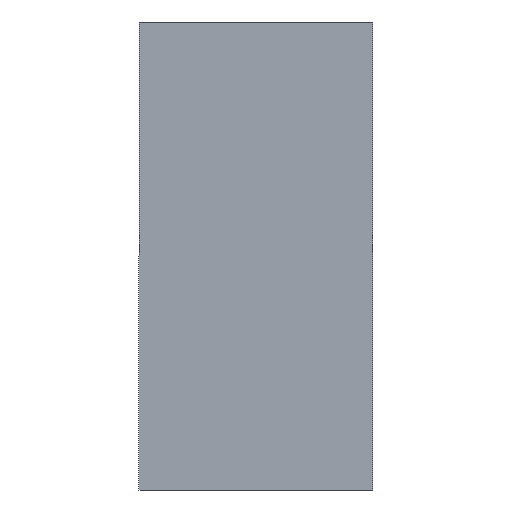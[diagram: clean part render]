
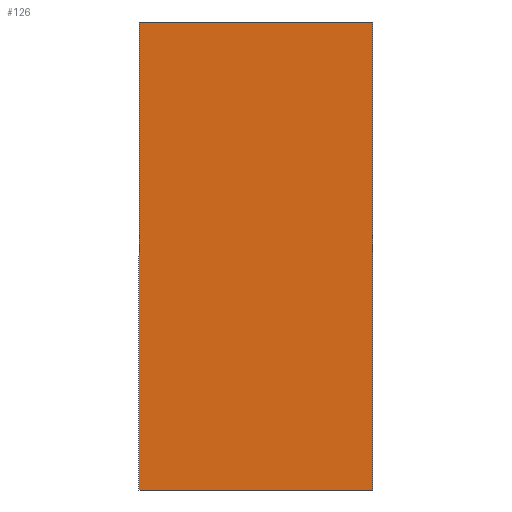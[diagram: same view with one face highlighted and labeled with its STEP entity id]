
A CAD part, front view. The second image highlights one B-rep face of the part: STEP entity #126.
In plain terms, the highlighted planar face has unit normal (0, -1, 0).
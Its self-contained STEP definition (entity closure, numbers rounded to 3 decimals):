
#19 = CARTESIAN_POINT ( 'NONE',  ( -12.7, -3.175, -25.4 ) ) ;
#24 = CARTESIAN_POINT ( 'NONE',  ( 12.7, -3.175, -25.4 ) ) ;
#29 = DIRECTION ( 'NONE',  ( 0., 1., 0. ) ) ;
#30 = VECTOR ( 'NONE', #66, 1000. ) ;
#38 = VERTEX_POINT ( 'NONE', #24 ) ;
#43 = EDGE_CURVE ( 'NONE', #144, #156, #130, .T. ) ;
#47 = DIRECTION ( 'NONE',  ( 0., 0., 1. ) ) ;
#52 = CARTESIAN_POINT ( 'NONE',  ( -12.7, -3.175, 25.4 ) ) ;
#66 = DIRECTION ( 'NONE',  ( -1., 0., 0. ) ) ;
#71 = ORIENTED_EDGE ( 'NONE', *, *, #206, .F. ) ;
#74 = FACE_OUTER_BOUND ( 'NONE', #96, .T. ) ;
#78 = VECTOR ( 'NONE', #143, 1000. ) ;
#81 = VECTOR ( 'NONE', #47, 1000. ) ;
#84 = PLANE ( 'NONE',  #183 ) ;
#85 = CARTESIAN_POINT ( 'NONE',  ( -12.7, -3.175, 25.4 ) ) ;
#96 = EDGE_LOOP ( 'NONE', ( #149, #232, #71, #197 ) ) ;
#112 = VECTOR ( 'NONE', #165, 1000. ) ;
#126 = ADVANCED_FACE ( 'NONE', ( #74 ), #84, .F. ) ;
#130 = LINE ( 'NONE', #85, #78 ) ;
#133 = LINE ( 'NONE', #178, #81 ) ;
#134 = CARTESIAN_POINT ( 'NONE',  ( 12.7, -3.175, -25.4 ) ) ;
#143 = DIRECTION ( 'NONE',  ( 1., 0., 0. ) ) ;
#144 = VERTEX_POINT ( 'NONE', #52 ) ;
#149 = ORIENTED_EDGE ( 'NONE', *, *, #245, .F. ) ;
#150 = CARTESIAN_POINT ( 'NONE',  ( -12.7, -3.175, -25.4 ) ) ;
#156 = VERTEX_POINT ( 'NONE', #234 ) ;
#162 = DIRECTION ( 'NONE',  ( 0., 0., 1. ) ) ;
#165 = DIRECTION ( 'NONE',  ( 0., 0., -1. ) ) ;
#178 = CARTESIAN_POINT ( 'NONE',  ( -12.7, -3.175, -25.4 ) ) ;
#183 = AXIS2_PLACEMENT_3D ( 'NONE', #184, #29, #162 ) ;
#184 = CARTESIAN_POINT ( 'NONE',  ( 0., -3.175, 0. ) ) ;
#197 = ORIENTED_EDGE ( 'NONE', *, *, #43, .F. ) ;
#202 = LINE ( 'NONE', #19, #30 ) ;
#206 = EDGE_CURVE ( 'NONE', #156, #38, #213, .T. ) ;
#213 = LINE ( 'NONE', #134, #112 ) ;
#230 = VERTEX_POINT ( 'NONE', #150 ) ;
#231 = EDGE_CURVE ( 'NONE', #38, #230, #202, .T. ) ;
#232 = ORIENTED_EDGE ( 'NONE', *, *, #231, .F. ) ;
#234 = CARTESIAN_POINT ( 'NONE',  ( 12.7, -3.175, 25.4 ) ) ;
#245 = EDGE_CURVE ( 'NONE', #230, #144, #133, .T. ) ;
